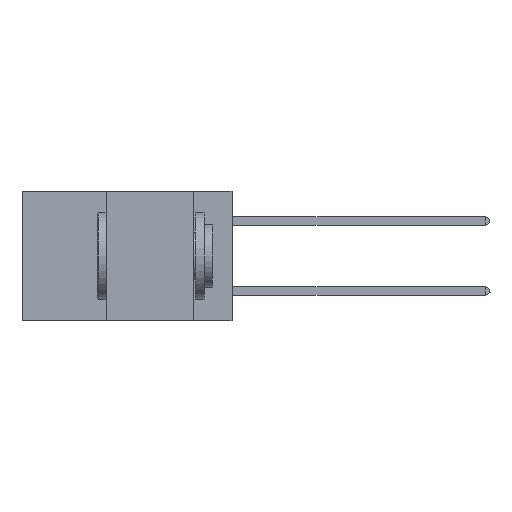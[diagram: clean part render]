
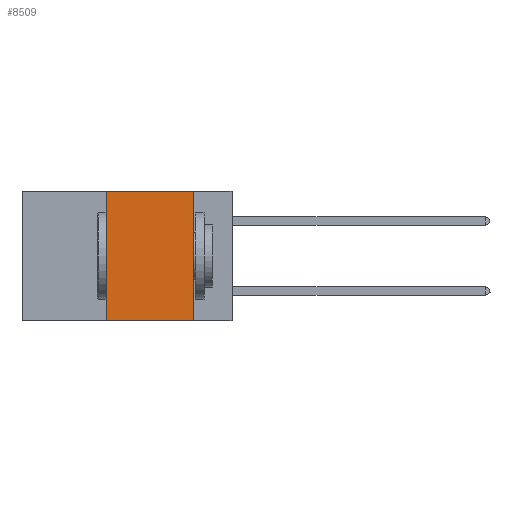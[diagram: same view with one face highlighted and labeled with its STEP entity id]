
A CAD part, left-side view. The second image highlights one B-rep face of the part: STEP entity #8509.
In plain terms, the highlighted planar face has unit normal (-1, 0, 0).
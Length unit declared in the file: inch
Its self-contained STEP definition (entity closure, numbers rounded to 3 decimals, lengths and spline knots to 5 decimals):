
#17 = ORIENTED_EDGE ( 'NONE', *, *, #10355, .F. ) ;
#1246 = ORIENTED_EDGE ( 'NONE', *, *, #6039, .F. ) ;
#1961 = AXIS2_PLACEMENT_3D ( 'NONE', #7443, #7348, #22311 ) ;
#3048 = VECTOR ( 'NONE', #3237, 39.37008 ) ;
#3124 = PLANE ( 'NONE',  #1961 ) ;
#3237 = DIRECTION ( 'NONE',  ( 0., -1., 0. ) ) ;
#3689 = DIRECTION ( 'NONE',  ( 0., 0., -1. ) ) ;
#3992 = LINE ( 'NONE', #11676, #21858 ) ;
#6039 = EDGE_CURVE ( 'NONE', #15610, #7302, #7299, .T. ) ;
#6106 = CARTESIAN_POINT ( 'NONE',  ( 0., 0.11, -0.37 ) ) ;
#7299 = LINE ( 'NONE', #15770, #3048 ) ;
#7302 = VERTEX_POINT ( 'NONE', #22186 ) ;
#7348 = DIRECTION ( 'NONE',  ( 1., 0., 0. ) ) ;
#7443 = CARTESIAN_POINT ( 'NONE',  ( 0., 0.6, 0. ) ) ;
#8509 = ADVANCED_FACE ( 'NONE', ( #16972 ), #3124, .F. ) ;
#10355 = EDGE_CURVE ( 'NONE', #22954, #15610, #18862, .T. ) ;
#10632 = DIRECTION ( 'NONE',  ( 0., 0., 1. ) ) ;
#11676 = CARTESIAN_POINT ( 'NONE',  ( 0., 0.6, -0.37 ) ) ;
#12384 = CARTESIAN_POINT ( 'NONE',  ( 0., 0.36, -0.37 ) ) ;
#14433 = CARTESIAN_POINT ( 'NONE',  ( 0., 0.36, 0. ) ) ;
#14488 = CARTESIAN_POINT ( 'NONE',  ( 0., 0.11, 0. ) ) ;
#14744 = EDGE_CURVE ( 'NONE', #7302, #16725, #24257, .T. ) ;
#15148 = ORIENTED_EDGE ( 'NONE', *, *, #17067, .T. ) ;
#15199 = VECTOR ( 'NONE', #10632, 39.37008 ) ;
#15610 = VERTEX_POINT ( 'NONE', #14433 ) ;
#15770 = CARTESIAN_POINT ( 'NONE',  ( 0., 0.6, 0. ) ) ;
#16725 = VERTEX_POINT ( 'NONE', #6106 ) ;
#16972 = FACE_OUTER_BOUND ( 'NONE', #21943, .T. ) ;
#17067 = EDGE_CURVE ( 'NONE', #22954, #16725, #3992, .T. ) ;
#18862 = LINE ( 'NONE', #22663, #15199 ) ;
#21268 = VECTOR ( 'NONE', #3689, 39.37008 ) ;
#21858 = VECTOR ( 'NONE', #24349, 39.37008 ) ;
#21943 = EDGE_LOOP ( 'NONE', ( #26740, #1246, #17, #15148 ) ) ;
#22186 = CARTESIAN_POINT ( 'NONE',  ( 0., 0.11, 0. ) ) ;
#22311 = DIRECTION ( 'NONE',  ( 0., 0., -1. ) ) ;
#22663 = CARTESIAN_POINT ( 'NONE',  ( 0., 0.36, 0. ) ) ;
#22954 = VERTEX_POINT ( 'NONE', #12384 ) ;
#24257 = LINE ( 'NONE', #14488, #21268 ) ;
#24349 = DIRECTION ( 'NONE',  ( 0., -1., 0. ) ) ;
#26740 = ORIENTED_EDGE ( 'NONE', *, *, #14744, .F. ) ;
